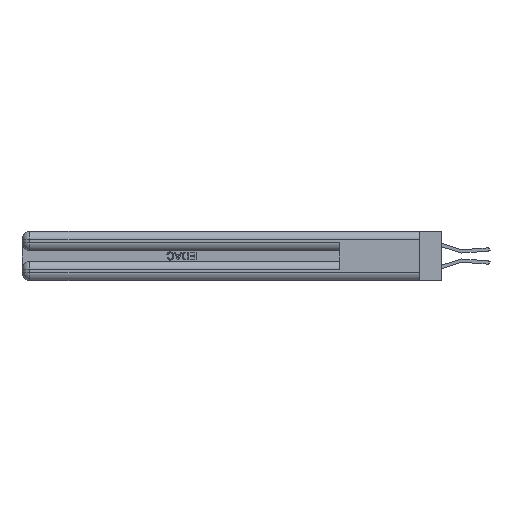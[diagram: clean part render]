
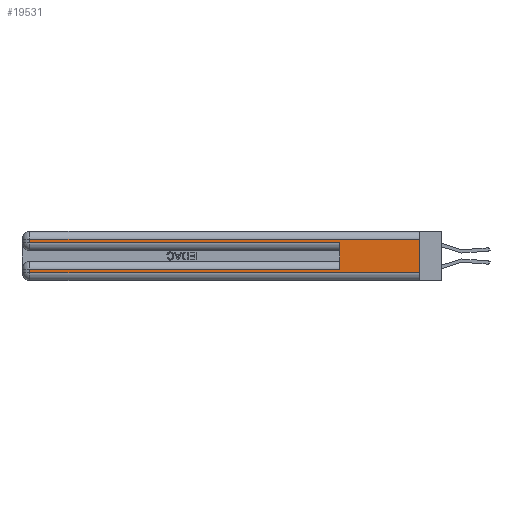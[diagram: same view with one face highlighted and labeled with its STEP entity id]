
A CAD part, left-side view. The second image highlights one B-rep face of the part: STEP entity #19531.
In plain terms, the highlighted planar face has unit normal (-1, 0, 0).
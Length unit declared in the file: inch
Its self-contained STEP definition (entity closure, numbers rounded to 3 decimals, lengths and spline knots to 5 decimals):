
#268 = EDGE_LOOP ( 'NONE', ( #38242, #5283, #19050, #32757, #39841, #3459, #35488, #38119 ) ) ;
#676 = CARTESIAN_POINT ( 'NONE',  ( 0., 2.94, 0.37 ) ) ;
#1020 = VERTEX_POINT ( 'NONE', #41991 ) ;
#1136 = VECTOR ( 'NONE', #11762, 39.37008 ) ;
#2653 = CARTESIAN_POINT ( 'NONE',  ( 0., 0., 0.085 ) ) ;
#3201 = EDGE_CURVE ( 'NONE', #41020, #19193, #14877, .T. ) ;
#3459 = ORIENTED_EDGE ( 'NONE', *, *, #25569, .T. ) ;
#3958 = LINE ( 'NONE', #676, #42503 ) ;
#4006 = LINE ( 'NONE', #6366, #30198 ) ;
#4433 = DIRECTION ( 'NONE',  ( 1., 0., 0. ) ) ;
#4701 = VECTOR ( 'NONE', #27699, 39.37008 ) ;
#5283 = ORIENTED_EDGE ( 'NONE', *, *, #12020, .T. ) ;
#6316 = VECTOR ( 'NONE', #9086, 39.37008 ) ;
#6366 = CARTESIAN_POINT ( 'NONE',  ( 0., 0.6, 0.145 ) ) ;
#6381 = CARTESIAN_POINT ( 'NONE',  ( 0., 0., 0.06 ) ) ;
#7502 = CARTESIAN_POINT ( 'NONE',  ( 0., 0., 0.37 ) ) ;
#7714 = DIRECTION ( 'NONE',  ( 0., 0., -1. ) ) ;
#9086 = DIRECTION ( 'NONE',  ( 0., 1., 0. ) ) ;
#9178 = LINE ( 'NONE', #21900, #1136 ) ;
#9743 = VERTEX_POINT ( 'NONE', #34644 ) ;
#11762 = DIRECTION ( 'NONE',  ( 0., 0., -1. ) ) ;
#11858 = VECTOR ( 'NONE', #31362, 39.37008 ) ;
#12020 = EDGE_CURVE ( 'NONE', #1020, #28780, #18246, .T. ) ;
#12079 = EDGE_CURVE ( 'NONE', #1020, #30897, #41708, .T. ) ;
#14877 = LINE ( 'NONE', #17295, #4701 ) ;
#17295 = CARTESIAN_POINT ( 'NONE',  ( 0., 0., 0.285 ) ) ;
#17838 = VERTEX_POINT ( 'NONE', #43628 ) ;
#18246 = LINE ( 'NONE', #40978, #41196 ) ;
#19050 = ORIENTED_EDGE ( 'NONE', *, *, #21732, .T. ) ;
#19193 = VERTEX_POINT ( 'NONE', #29041 ) ;
#19531 = ADVANCED_FACE ( 'NONE', ( #40905 ), #42393, .F. ) ;
#20607 = AXIS2_PLACEMENT_3D ( 'NONE', #25477, #4433, #32646 ) ;
#21732 = EDGE_CURVE ( 'NONE', #28780, #41020, #9178, .T. ) ;
#21900 = CARTESIAN_POINT ( 'NONE',  ( 0., 2.94, 0.37 ) ) ;
#22088 = EDGE_CURVE ( 'NONE', #9743, #30897, #28885, .T. ) ;
#25477 = CARTESIAN_POINT ( 'NONE',  ( 0., 0., 0.37 ) ) ;
#25569 = EDGE_CURVE ( 'NONE', #42959, #17838, #25575, .T. ) ;
#25575 = LINE ( 'NONE', #2653, #6316 ) ;
#25611 = CARTESIAN_POINT ( 'NONE',  ( 0., 2.94, 0.285 ) ) ;
#25983 = CARTESIAN_POINT ( 'NONE',  ( 0., 2.94, 0.31 ) ) ;
#27699 = DIRECTION ( 'NONE',  ( 0., -1., 0. ) ) ;
#28243 = EDGE_CURVE ( 'NONE', #42959, #19193, #4006, .T. ) ;
#28482 = EDGE_CURVE ( 'NONE', #17838, #9743, #3958, .T. ) ;
#28780 = VERTEX_POINT ( 'NONE', #25983 ) ;
#28885 = LINE ( 'NONE', #35943, #40658 ) ;
#29041 = CARTESIAN_POINT ( 'NONE',  ( 0., 0.6, 0.285 ) ) ;
#30198 = VECTOR ( 'NONE', #40450, 39.37008 ) ;
#30218 = DIRECTION ( 'NONE',  ( 0., 1., 0. ) ) ;
#30897 = VERTEX_POINT ( 'NONE', #6381 ) ;
#31362 = DIRECTION ( 'NONE',  ( 0., 0., -1. ) ) ;
#32646 = DIRECTION ( 'NONE',  ( 0., 0., -1. ) ) ;
#32757 = ORIENTED_EDGE ( 'NONE', *, *, #3201, .T. ) ;
#32779 = CARTESIAN_POINT ( 'NONE',  ( 0., 0.6, 0.085 ) ) ;
#34644 = CARTESIAN_POINT ( 'NONE',  ( 0., 2.94, 0.06 ) ) ;
#35488 = ORIENTED_EDGE ( 'NONE', *, *, #28482, .T. ) ;
#35943 = CARTESIAN_POINT ( 'NONE',  ( 0., 0., 0.06 ) ) ;
#38119 = ORIENTED_EDGE ( 'NONE', *, *, #22088, .T. ) ;
#38242 = ORIENTED_EDGE ( 'NONE', *, *, #12079, .F. ) ;
#39526 = DIRECTION ( 'NONE',  ( 0., -1., 0. ) ) ;
#39841 = ORIENTED_EDGE ( 'NONE', *, *, #28243, .F. ) ;
#40450 = DIRECTION ( 'NONE',  ( 0., 0., 1. ) ) ;
#40658 = VECTOR ( 'NONE', #39526, 39.37008 ) ;
#40905 = FACE_OUTER_BOUND ( 'NONE', #268, .T. ) ;
#40978 = CARTESIAN_POINT ( 'NONE',  ( 0., 0., 0.31 ) ) ;
#41020 = VERTEX_POINT ( 'NONE', #25611 ) ;
#41196 = VECTOR ( 'NONE', #30218, 39.37008 ) ;
#41708 = LINE ( 'NONE', #7502, #11858 ) ;
#41991 = CARTESIAN_POINT ( 'NONE',  ( 0., 0., 0.31 ) ) ;
#42393 = PLANE ( 'NONE',  #20607 ) ;
#42503 = VECTOR ( 'NONE', #7714, 39.37008 ) ;
#42959 = VERTEX_POINT ( 'NONE', #32779 ) ;
#43628 = CARTESIAN_POINT ( 'NONE',  ( 0., 2.94, 0.085 ) ) ;
